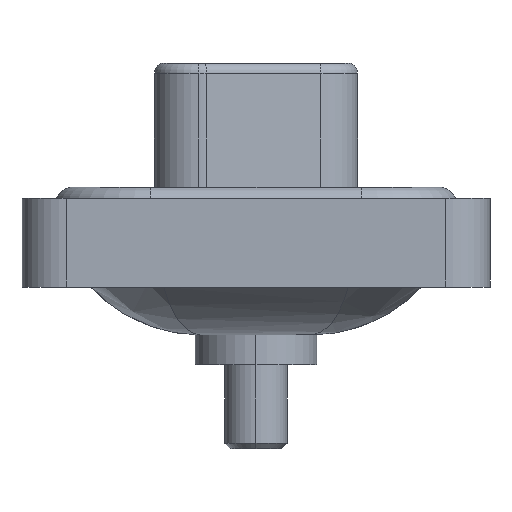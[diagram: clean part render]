
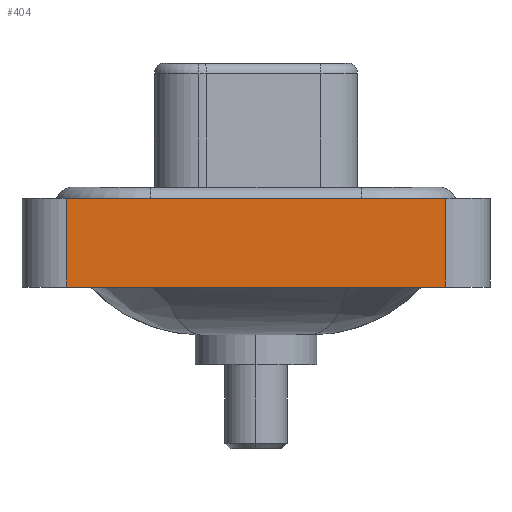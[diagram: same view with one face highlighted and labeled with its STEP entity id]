
A CAD part, left-side view. The second image highlights one B-rep face of the part: STEP entity #404.
In plain terms, the highlighted planar face has unit normal (-1, 0, 0).
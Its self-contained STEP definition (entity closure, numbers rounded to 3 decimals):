
#207 = CARTESIAN_POINT ( 'NONE',  ( -7.25, -8.55, 0.4 ) ) ;
#404 = ADVANCED_FACE ( 'NONE', ( #6424 ), #786, .T. ) ;
#786 = PLANE ( 'NONE',  #6535 ) ;
#1331 = VERTEX_POINT ( 'NONE', #14392 ) ;
#1492 = EDGE_CURVE ( 'NONE', #7012, #1331, #13787, .T. ) ;
#1545 = DIRECTION ( 'NONE',  ( 0., -1., 0. ) ) ;
#2269 = DIRECTION ( 'NONE',  ( 0., 0., 1. ) ) ;
#2512 = CARTESIAN_POINT ( 'NONE',  ( -7.25, -8.55, -3.6 ) ) ;
#2667 = CARTESIAN_POINT ( 'NONE',  ( -7.25, 8.55, -3.6 ) ) ;
#2708 = EDGE_CURVE ( 'NONE', #12786, #1331, #6476, .T. ) ;
#3650 = CARTESIAN_POINT ( 'NONE',  ( -7.25, -8.55, -3.6 ) ) ;
#4177 = LINE ( 'NONE', #11053, #7529 ) ;
#4345 = CARTESIAN_POINT ( 'NONE',  ( -7.25, -8.55, -3.6 ) ) ;
#4445 = EDGE_CURVE ( 'NONE', #5099, #12786, #17452, .T. ) ;
#4740 = DIRECTION ( 'NONE',  ( -1., 0., 0. ) ) ;
#5099 = VERTEX_POINT ( 'NONE', #2667 ) ;
#6424 = FACE_OUTER_BOUND ( 'NONE', #9958, .T. ) ;
#6476 = LINE ( 'NONE', #11930, #7231 ) ;
#6535 = AXIS2_PLACEMENT_3D ( 'NONE', #3650, #4740, #11619 ) ;
#6570 = CARTESIAN_POINT ( 'NONE',  ( -7.25, 8.55, 0.4 ) ) ;
#6602 = ORIENTED_EDGE ( 'NONE', *, *, #1492, .F. ) ;
#7012 = VERTEX_POINT ( 'NONE', #6570 ) ;
#7231 = VECTOR ( 'NONE', #2269, 1000. ) ;
#7262 = VECTOR ( 'NONE', #13427, 1000. ) ;
#7529 = VECTOR ( 'NONE', #13896, 1000. ) ;
#8384 = VECTOR ( 'NONE', #1545, 1000. ) ;
#9958 = EDGE_LOOP ( 'NONE', ( #16435, #6602, #12197, #16308 ) ) ;
#11053 = CARTESIAN_POINT ( 'NONE',  ( -7.25, 8.55, -3.6 ) ) ;
#11619 = DIRECTION ( 'NONE',  ( 0., 0., 1. ) ) ;
#11930 = CARTESIAN_POINT ( 'NONE',  ( -7.25, -8.55, -3.6 ) ) ;
#12197 = ORIENTED_EDGE ( 'NONE', *, *, #12730, .F. ) ;
#12730 = EDGE_CURVE ( 'NONE', #5099, #7012, #4177, .T. ) ;
#12786 = VERTEX_POINT ( 'NONE', #4345 ) ;
#13427 = DIRECTION ( 'NONE',  ( 0., -1., 0. ) ) ;
#13787 = LINE ( 'NONE', #207, #8384 ) ;
#13896 = DIRECTION ( 'NONE',  ( 0., 0., 1. ) ) ;
#14392 = CARTESIAN_POINT ( 'NONE',  ( -7.25, -8.55, 0.4 ) ) ;
#16308 = ORIENTED_EDGE ( 'NONE', *, *, #4445, .T. ) ;
#16435 = ORIENTED_EDGE ( 'NONE', *, *, #2708, .T. ) ;
#17452 = LINE ( 'NONE', #2512, #7262 ) ;
